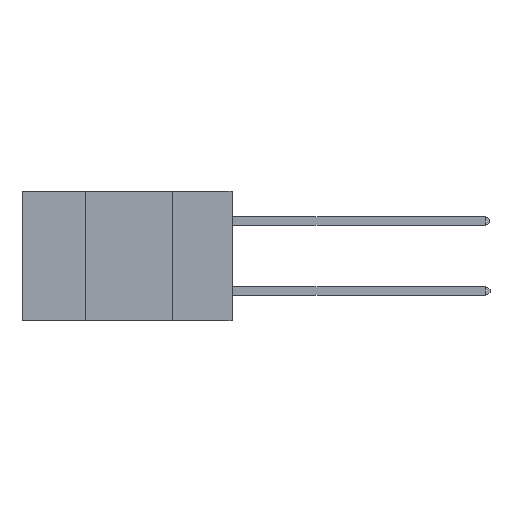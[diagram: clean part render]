
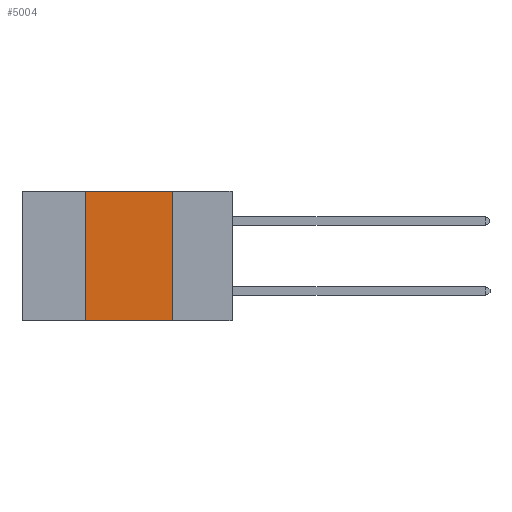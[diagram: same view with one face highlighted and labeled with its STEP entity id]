
A CAD part, left-side view. The second image highlights one B-rep face of the part: STEP entity #5004.
In plain terms, the highlighted planar face has unit normal (-1, 0, 0).
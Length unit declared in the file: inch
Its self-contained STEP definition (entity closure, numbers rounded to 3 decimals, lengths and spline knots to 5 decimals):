
#500 = VERTEX_POINT ( 'NONE', #1600 ) ;
#1600 = CARTESIAN_POINT ( 'NONE',  ( 0., 0.42, 0. ) ) ;
#1745 = AXIS2_PLACEMENT_3D ( 'NONE', #19920, #9232, #21703 ) ;
#2634 = VECTOR ( 'NONE', #8754, 39.37008 ) ;
#4104 = VERTEX_POINT ( 'NONE', #10348 ) ;
#5004 = ADVANCED_FACE ( 'NONE', ( #17763 ), #16314, .F. ) ;
#5150 = VECTOR ( 'NONE', #22269, 39.37008 ) ;
#5220 = ORIENTED_EDGE ( 'NONE', *, *, #19553, .F. ) ;
#5610 = ORIENTED_EDGE ( 'NONE', *, *, #21992, .F. ) ;
#7677 = VERTEX_POINT ( 'NONE', #10781 ) ;
#7711 = CARTESIAN_POINT ( 'NONE',  ( 0., 0.17, 0. ) ) ;
#8452 = VECTOR ( 'NONE', #10988, 39.37008 ) ;
#8754 = DIRECTION ( 'NONE',  ( 0., -1., 0. ) ) ;
#9208 = CARTESIAN_POINT ( 'NONE',  ( 0., 0.6, -0.37 ) ) ;
#9232 = DIRECTION ( 'NONE',  ( 1., 0., 0. ) ) ;
#10348 = CARTESIAN_POINT ( 'NONE',  ( 0., 0.17, -0.37 ) ) ;
#10781 = CARTESIAN_POINT ( 'NONE',  ( 0., 0.42, -0.37 ) ) ;
#10988 = DIRECTION ( 'NONE',  ( 0., -1., 0. ) ) ;
#11284 = DIRECTION ( 'NONE',  ( 0., 0., -1. ) ) ;
#12396 = EDGE_CURVE ( 'NONE', #12817, #4104, #16001, .T. ) ;
#12458 = CARTESIAN_POINT ( 'NONE',  ( 0., 0.17, 0. ) ) ;
#12817 = VERTEX_POINT ( 'NONE', #12458 ) ;
#13622 = EDGE_CURVE ( 'NONE', #7677, #4104, #17933, .T. ) ;
#14843 = EDGE_LOOP ( 'NONE', ( #15107, #5610, #5220, #20403 ) ) ;
#15107 = ORIENTED_EDGE ( 'NONE', *, *, #12396, .F. ) ;
#16001 = LINE ( 'NONE', #7711, #19636 ) ;
#16314 = PLANE ( 'NONE',  #1745 ) ;
#17763 = FACE_OUTER_BOUND ( 'NONE', #14843, .T. ) ;
#17933 = LINE ( 'NONE', #9208, #8452 ) ;
#19417 = LINE ( 'NONE', #22196, #5150 ) ;
#19553 = EDGE_CURVE ( 'NONE', #7677, #500, #19417, .T. ) ;
#19636 = VECTOR ( 'NONE', #11284, 39.37008 ) ;
#19920 = CARTESIAN_POINT ( 'NONE',  ( 0., 0.6, 0. ) ) ;
#20403 = ORIENTED_EDGE ( 'NONE', *, *, #13622, .T. ) ;
#21217 = CARTESIAN_POINT ( 'NONE',  ( 0., 0.6, 0. ) ) ;
#21223 = LINE ( 'NONE', #21217, #2634 ) ;
#21703 = DIRECTION ( 'NONE',  ( 0., 0., -1. ) ) ;
#21992 = EDGE_CURVE ( 'NONE', #500, #12817, #21223, .T. ) ;
#22196 = CARTESIAN_POINT ( 'NONE',  ( 0., 0.42, 0. ) ) ;
#22269 = DIRECTION ( 'NONE',  ( 0., 0., 1. ) ) ;
